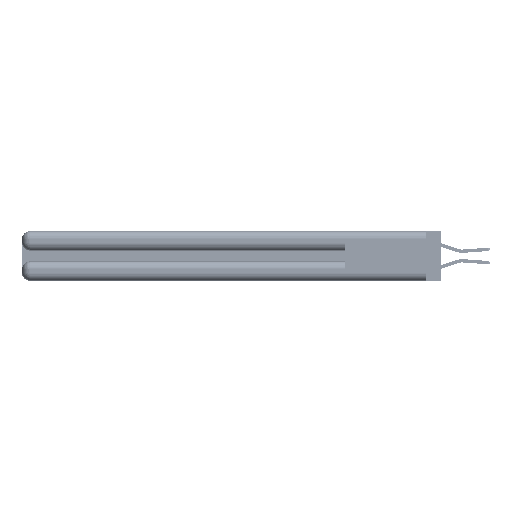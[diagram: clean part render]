
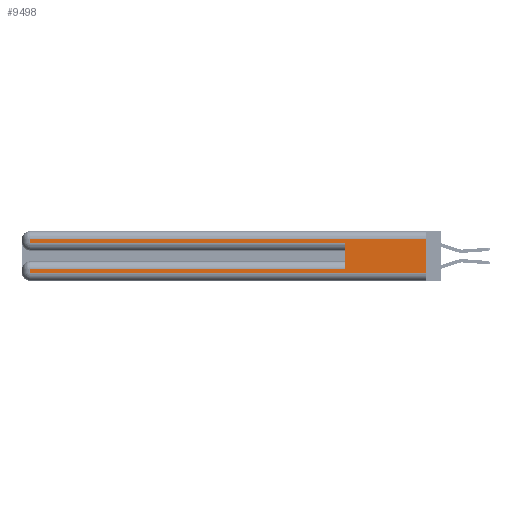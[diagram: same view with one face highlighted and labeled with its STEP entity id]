
A CAD part, left-side view. The second image highlights one B-rep face of the part: STEP entity #9498.
In plain terms, the highlighted planar face has unit normal (-1, 0, 0).
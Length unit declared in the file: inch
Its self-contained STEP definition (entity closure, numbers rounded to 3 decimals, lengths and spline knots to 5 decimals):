
#1118 = ORIENTED_EDGE ( 'NONE', *, *, #7931, .T. ) ;
#1176 = FACE_OUTER_BOUND ( 'NONE', #23594, .T. ) ;
#3177 = DIRECTION ( 'NONE',  ( 0., -1., 0. ) ) ;
#3220 = CARTESIAN_POINT ( 'NONE',  ( 0., 0.6, 0.145 ) ) ;
#4180 = CARTESIAN_POINT ( 'NONE',  ( 0., 0., 0.37 ) ) ;
#4369 = CARTESIAN_POINT ( 'NONE',  ( 0., 0., 0.06 ) ) ;
#4618 = LINE ( 'NONE', #24975, #13857 ) ;
#5437 = ORIENTED_EDGE ( 'NONE', *, *, #17061, .T. ) ;
#6532 = EDGE_CURVE ( 'NONE', #53232, #15403, #32560, .T. ) ;
#7306 = LINE ( 'NONE', #3220, #16518 ) ;
#7822 = DIRECTION ( 'NONE',  ( 0., 0., 1. ) ) ;
#7931 = EDGE_CURVE ( 'NONE', #52204, #53232, #9929, .T. ) ;
#8683 = VECTOR ( 'NONE', #3177, 39.37008 ) ;
#9155 = EDGE_CURVE ( 'NONE', #26839, #15403, #30191, .T. ) ;
#9498 = ADVANCED_FACE ( 'NONE', ( #1176 ), #10737, .F. ) ;
#9929 = LINE ( 'NONE', #43637, #55879 ) ;
#10522 = EDGE_CURVE ( 'NONE', #49857, #52242, #13812, .T. ) ;
#10737 = PLANE ( 'NONE',  #52591 ) ;
#12152 = VECTOR ( 'NONE', #55739, 39.37008 ) ;
#12895 = ORIENTED_EDGE ( 'NONE', *, *, #45575, .F. ) ;
#13812 = LINE ( 'NONE', #22057, #36188 ) ;
#13857 = VECTOR ( 'NONE', #47271, 39.37008 ) ;
#15285 = DIRECTION ( 'NONE',  ( 0., 0., -1. ) ) ;
#15403 = VERTEX_POINT ( 'NONE', #4369 ) ;
#15740 = CARTESIAN_POINT ( 'NONE',  ( 0., 0., 0.285 ) ) ;
#15866 = CARTESIAN_POINT ( 'NONE',  ( 0., 0., 0.31 ) ) ;
#16026 = ORIENTED_EDGE ( 'NONE', *, *, #6532, .T. ) ;
#16518 = VECTOR ( 'NONE', #7822, 39.37008 ) ;
#17061 = EDGE_CURVE ( 'NONE', #52851, #52204, #4618, .T. ) ;
#17669 = EDGE_CURVE ( 'NONE', #26839, #49857, #42451, .T. ) ;
#22057 = CARTESIAN_POINT ( 'NONE',  ( 0., 2.94, 0.37 ) ) ;
#23594 = EDGE_LOOP ( 'NONE', ( #56991, #34952, #28000, #28776, #12895, #5437, #1118, #16026 ) ) ;
#24975 = CARTESIAN_POINT ( 'NONE',  ( 0., 0., 0.085 ) ) ;
#25171 = CARTESIAN_POINT ( 'NONE',  ( 0., 0., 0.31 ) ) ;
#25952 = DIRECTION ( 'NONE',  ( 0., 0., -1. ) ) ;
#26566 = DIRECTION ( 'NONE',  ( 0., 0., -1. ) ) ;
#26839 = VERTEX_POINT ( 'NONE', #25171 ) ;
#28000 = ORIENTED_EDGE ( 'NONE', *, *, #10522, .T. ) ;
#28776 = ORIENTED_EDGE ( 'NONE', *, *, #29130, .T. ) ;
#29130 = EDGE_CURVE ( 'NONE', #52242, #39985, #47726, .T. ) ;
#30191 = LINE ( 'NONE', #4180, #41986 ) ;
#32560 = LINE ( 'NONE', #43398, #8683 ) ;
#34952 = ORIENTED_EDGE ( 'NONE', *, *, #17669, .T. ) ;
#35618 = DIRECTION ( 'NONE',  ( 0., 0., -1. ) ) ;
#36188 = VECTOR ( 'NONE', #26566, 39.37008 ) ;
#37766 = CARTESIAN_POINT ( 'NONE',  ( 0., 2.94, 0.31 ) ) ;
#39985 = VERTEX_POINT ( 'NONE', #56523 ) ;
#41945 = CARTESIAN_POINT ( 'NONE',  ( 0., 0.6, 0.085 ) ) ;
#41986 = VECTOR ( 'NONE', #35618, 39.37008 ) ;
#42015 = DIRECTION ( 'NONE',  ( 1., 0., 0. ) ) ;
#42451 = LINE ( 'NONE', #15866, #52763 ) ;
#43398 = CARTESIAN_POINT ( 'NONE',  ( 0., 0., 0.06 ) ) ;
#43637 = CARTESIAN_POINT ( 'NONE',  ( 0., 2.94, 0.37 ) ) ;
#44044 = CARTESIAN_POINT ( 'NONE',  ( 0., 2.94, 0.06 ) ) ;
#45575 = EDGE_CURVE ( 'NONE', #52851, #39985, #7306, .T. ) ;
#46044 = CARTESIAN_POINT ( 'NONE',  ( 0., 2.94, 0.085 ) ) ;
#46238 = CARTESIAN_POINT ( 'NONE',  ( 0., 0., 0.37 ) ) ;
#47271 = DIRECTION ( 'NONE',  ( 0., 1., 0. ) ) ;
#47726 = LINE ( 'NONE', #15740, #12152 ) ;
#49857 = VERTEX_POINT ( 'NONE', #37766 ) ;
#50671 = CARTESIAN_POINT ( 'NONE',  ( 0., 2.94, 0.285 ) ) ;
#51422 = DIRECTION ( 'NONE',  ( 0., 1., 0. ) ) ;
#52204 = VERTEX_POINT ( 'NONE', #46044 ) ;
#52242 = VERTEX_POINT ( 'NONE', #50671 ) ;
#52591 = AXIS2_PLACEMENT_3D ( 'NONE', #46238, #42015, #15285 ) ;
#52763 = VECTOR ( 'NONE', #51422, 39.37008 ) ;
#52851 = VERTEX_POINT ( 'NONE', #41945 ) ;
#53232 = VERTEX_POINT ( 'NONE', #44044 ) ;
#55739 = DIRECTION ( 'NONE',  ( 0., -1., 0. ) ) ;
#55879 = VECTOR ( 'NONE', #25952, 39.37008 ) ;
#56523 = CARTESIAN_POINT ( 'NONE',  ( 0., 0.6, 0.285 ) ) ;
#56991 = ORIENTED_EDGE ( 'NONE', *, *, #9155, .F. ) ;
